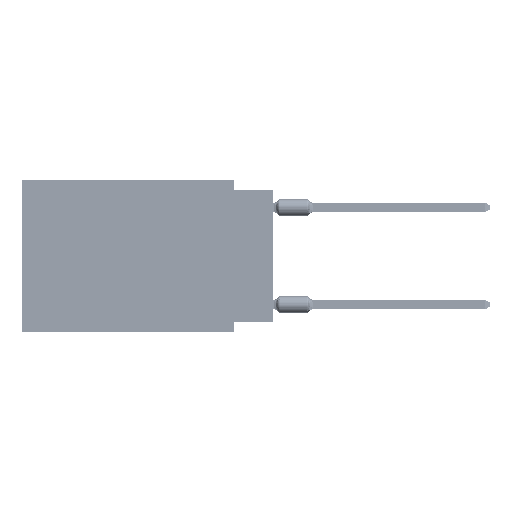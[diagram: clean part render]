
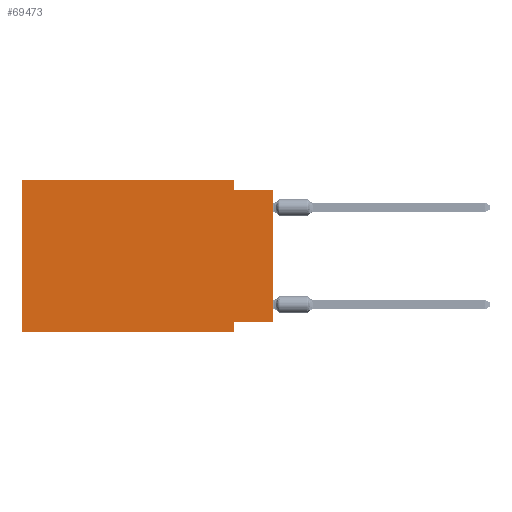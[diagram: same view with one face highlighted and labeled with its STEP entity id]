
A CAD part, left-side view. The second image highlights one B-rep face of the part: STEP entity #69473.
In plain terms, the highlighted planar face has unit normal (-1, 0, 0).
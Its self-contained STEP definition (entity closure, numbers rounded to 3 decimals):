
#381 = CARTESIAN_POINT ( 'NONE',  ( 0., 2.54, -0.635 ) ) ;
#3484 = EDGE_CURVE ( 'NONE', #22013, #41936, #10785, .T. ) ;
#3961 = VECTOR ( 'NONE', #6465, 1000. ) ;
#4547 = VECTOR ( 'NONE', #62877, 1000. ) ;
#4614 = VERTEX_POINT ( 'NONE', #13108 ) ;
#5744 = CARTESIAN_POINT ( 'NONE',  ( 0., 0., -0.635 ) ) ;
#6383 = ORIENTED_EDGE ( 'NONE', *, *, #35649, .F. ) ;
#6465 = DIRECTION ( 'NONE',  ( 0., 0., -1. ) ) ;
#6544 = VECTOR ( 'NONE', #24274, 1000. ) ;
#7386 = ORIENTED_EDGE ( 'NONE', *, *, #23786, .T. ) ;
#9565 = DIRECTION ( 'NONE',  ( 1., 0., 0. ) ) ;
#10785 = LINE ( 'NONE', #36827, #4547 ) ;
#13108 = CARTESIAN_POINT ( 'NONE',  ( 0., 16.383, 0. ) ) ;
#19276 = LINE ( 'NONE', #27401, #3961 ) ;
#21003 = DIRECTION ( 'NONE',  ( 0., 0., 1. ) ) ;
#21158 = CARTESIAN_POINT ( 'NONE',  ( 0., 0., -9.271 ) ) ;
#21963 = CARTESIAN_POINT ( 'NONE',  ( 0., 16.383, 0. ) ) ;
#22013 = VERTEX_POINT ( 'NONE', #381 ) ;
#23745 = ORIENTED_EDGE ( 'NONE', *, *, #33494, .T. ) ;
#23786 = EDGE_CURVE ( 'NONE', #55017, #69061, #61792, .T. ) ;
#24164 = CARTESIAN_POINT ( 'NONE',  ( 0., 16.383, 0. ) ) ;
#24274 = DIRECTION ( 'NONE',  ( 0., 0., -1. ) ) ;
#24707 = LINE ( 'NONE', #63137, #6544 ) ;
#25021 = LINE ( 'NONE', #24164, #51534 ) ;
#26001 = ORIENTED_EDGE ( 'NONE', *, *, #3484, .F. ) ;
#27401 = CARTESIAN_POINT ( 'NONE',  ( 0., 2.54, -9.906 ) ) ;
#28423 = ORIENTED_EDGE ( 'NONE', *, *, #83227, .F. ) ;
#29190 = FACE_OUTER_BOUND ( 'NONE', #31719, .T. ) ;
#30668 = VERTEX_POINT ( 'NONE', #58908 ) ;
#31719 = EDGE_LOOP ( 'NONE', ( #23745, #26001, #57235, #6383, #28423, #7386, #63278, #78742 ) ) ;
#33494 = EDGE_CURVE ( 'NONE', #66120, #41936, #40214, .T. ) ;
#34762 = PLANE ( 'NONE',  #42980 ) ;
#35249 = EDGE_CURVE ( 'NONE', #30668, #22013, #24707, .T. ) ;
#35319 = CARTESIAN_POINT ( 'NONE',  ( 0., 0., -9.271 ) ) ;
#35649 = EDGE_CURVE ( 'NONE', #4614, #30668, #25021, .T. ) ;
#36827 = CARTESIAN_POINT ( 'NONE',  ( 0., 0., -0.635 ) ) ;
#40214 = LINE ( 'NONE', #66270, #71767 ) ;
#40727 = EDGE_CURVE ( 'NONE', #42572, #69061, #19276, .T. ) ;
#41936 = VERTEX_POINT ( 'NONE', #5744 ) ;
#42208 = CARTESIAN_POINT ( 'NONE',  ( 0., 2.54, -9.906 ) ) ;
#42572 = VERTEX_POINT ( 'NONE', #69094 ) ;
#42980 = AXIS2_PLACEMENT_3D ( 'NONE', #21963, #9565, #80472 ) ;
#51534 = VECTOR ( 'NONE', #70689, 1000. ) ;
#52435 = VECTOR ( 'NONE', #80914, 1000. ) ;
#55017 = VERTEX_POINT ( 'NONE', #70447 ) ;
#55378 = CARTESIAN_POINT ( 'NONE',  ( 0., 16.383, -9.906 ) ) ;
#57048 = DIRECTION ( 'NONE',  ( 0., -1., 0. ) ) ;
#57235 = ORIENTED_EDGE ( 'NONE', *, *, #35249, .F. ) ;
#58908 = CARTESIAN_POINT ( 'NONE',  ( 0., 2.54, 0. ) ) ;
#60022 = LINE ( 'NONE', #21158, #79318 ) ;
#61792 = LINE ( 'NONE', #55378, #77177 ) ;
#62877 = DIRECTION ( 'NONE',  ( 0., -1., 0. ) ) ;
#63137 = CARTESIAN_POINT ( 'NONE',  ( 0., 2.54, 0. ) ) ;
#63278 = ORIENTED_EDGE ( 'NONE', *, *, #40727, .F. ) ;
#66120 = VERTEX_POINT ( 'NONE', #35319 ) ;
#66270 = CARTESIAN_POINT ( 'NONE',  ( 0., 0., 0. ) ) ;
#67573 = EDGE_CURVE ( 'NONE', #66120, #42572, #60022, .T. ) ;
#67682 = LINE ( 'NONE', #81754, #52435 ) ;
#69061 = VERTEX_POINT ( 'NONE', #42208 ) ;
#69094 = CARTESIAN_POINT ( 'NONE',  ( 0., 2.54, -9.271 ) ) ;
#69473 = ADVANCED_FACE ( 'NONE', ( #29190 ), #34762, .F. ) ;
#70447 = CARTESIAN_POINT ( 'NONE',  ( 0., 16.383, -9.906 ) ) ;
#70689 = DIRECTION ( 'NONE',  ( 0., -1., 0. ) ) ;
#71767 = VECTOR ( 'NONE', #21003, 1000. ) ;
#77177 = VECTOR ( 'NONE', #57048, 1000. ) ;
#78742 = ORIENTED_EDGE ( 'NONE', *, *, #67573, .F. ) ;
#78786 = DIRECTION ( 'NONE',  ( 0., 1., 0. ) ) ;
#79318 = VECTOR ( 'NONE', #78786, 1000. ) ;
#80472 = DIRECTION ( 'NONE',  ( 0., 0., -1. ) ) ;
#80914 = DIRECTION ( 'NONE',  ( 0., 0., 1. ) ) ;
#81754 = CARTESIAN_POINT ( 'NONE',  ( 0., 16.383, 0. ) ) ;
#83227 = EDGE_CURVE ( 'NONE', #55017, #4614, #67682, .T. ) ;
